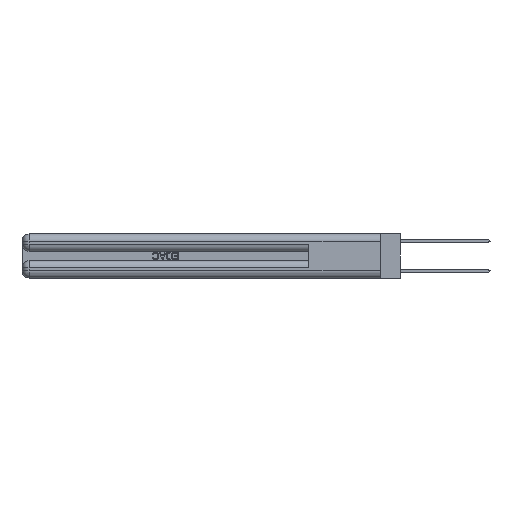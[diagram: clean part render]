
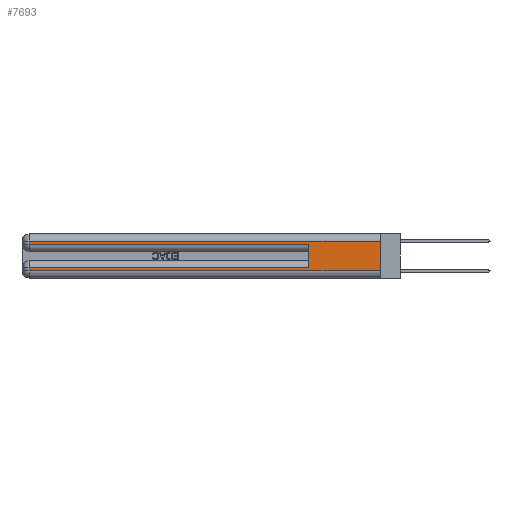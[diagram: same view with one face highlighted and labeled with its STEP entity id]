
A CAD part, left-side view. The second image highlights one B-rep face of the part: STEP entity #7693.
In plain terms, the highlighted planar face has unit normal (-1, 0, 0).
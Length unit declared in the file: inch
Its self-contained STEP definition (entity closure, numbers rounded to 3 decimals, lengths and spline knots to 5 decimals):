
#2025 = DIRECTION ( 'NONE',  ( 0., 0., -1. ) ) ;
#2323 = ORIENTED_EDGE ( 'NONE', *, *, #17587, .T. ) ;
#2801 = VECTOR ( 'NONE', #30167, 39.37008 ) ;
#4082 = CARTESIAN_POINT ( 'NONE',  ( 0., 0., 0.37 ) ) ;
#4154 = LINE ( 'NONE', #16316, #6959 ) ;
#4185 = CARTESIAN_POINT ( 'NONE',  ( 0., 2.94, 0.31 ) ) ;
#5009 = CARTESIAN_POINT ( 'NONE',  ( 0., 0., 0.31 ) ) ;
#6556 = LINE ( 'NONE', #8616, #17655 ) ;
#6946 = CARTESIAN_POINT ( 'NONE',  ( 0., 2.94, 0.37 ) ) ;
#6959 = VECTOR ( 'NONE', #13792, 39.37008 ) ;
#7693 = ADVANCED_FACE ( 'NONE', ( #28511 ), #28042, .F. ) ;
#8075 = DIRECTION ( 'NONE',  ( 0., -1., 0. ) ) ;
#8616 = CARTESIAN_POINT ( 'NONE',  ( 0., 0., 0.085 ) ) ;
#8637 = VECTOR ( 'NONE', #30842, 39.37008 ) ;
#9933 = CARTESIAN_POINT ( 'NONE',  ( 0., 0., 0.37 ) ) ;
#10361 = EDGE_LOOP ( 'NONE', ( #27957, #25769, #2323, #22479, #22251, #14810, #10801, #22275 ) ) ;
#10647 = VERTEX_POINT ( 'NONE', #10751 ) ;
#10662 = CARTESIAN_POINT ( 'NONE',  ( 0., 0.6, 0.285 ) ) ;
#10751 = CARTESIAN_POINT ( 'NONE',  ( 0., 0., 0.06 ) ) ;
#10801 = ORIENTED_EDGE ( 'NONE', *, *, #30165, .T. ) ;
#10812 = LINE ( 'NONE', #22941, #2801 ) ;
#12422 = VECTOR ( 'NONE', #28984, 39.37008 ) ;
#12439 = EDGE_CURVE ( 'NONE', #19086, #18914, #20362, .T. ) ;
#12474 = VERTEX_POINT ( 'NONE', #21292 ) ;
#12610 = DIRECTION ( 'NONE',  ( 1., 0., 0. ) ) ;
#13792 = DIRECTION ( 'NONE',  ( 0., 1., 0. ) ) ;
#14315 = EDGE_CURVE ( 'NONE', #18334, #10647, #14336, .T. ) ;
#14336 = LINE ( 'NONE', #24078, #14545 ) ;
#14545 = VECTOR ( 'NONE', #29401, 39.37008 ) ;
#14810 = ORIENTED_EDGE ( 'NONE', *, *, #25008, .T. ) ;
#15724 = VERTEX_POINT ( 'NONE', #5009 ) ;
#16025 = CARTESIAN_POINT ( 'NONE',  ( 0., 2.94, 0.285 ) ) ;
#16177 = DIRECTION ( 'NONE',  ( 0., 1., 0. ) ) ;
#16316 = CARTESIAN_POINT ( 'NONE',  ( 0., 0., 0.31 ) ) ;
#16795 = VERTEX_POINT ( 'NONE', #28550 ) ;
#17587 = EDGE_CURVE ( 'NONE', #19138, #19086, #23912, .T. ) ;
#17655 = VECTOR ( 'NONE', #16177, 39.37008 ) ;
#18334 = VERTEX_POINT ( 'NONE', #30897 ) ;
#18914 = VERTEX_POINT ( 'NONE', #10662 ) ;
#19086 = VERTEX_POINT ( 'NONE', #16025 ) ;
#19138 = VERTEX_POINT ( 'NONE', #4185 ) ;
#19347 = CARTESIAN_POINT ( 'NONE',  ( 0., 2.94, 0.37 ) ) ;
#19397 = LINE ( 'NONE', #6946, #12422 ) ;
#19762 = VECTOR ( 'NONE', #8075, 39.37008 ) ;
#20362 = LINE ( 'NONE', #29636, #19762 ) ;
#21292 = CARTESIAN_POINT ( 'NONE',  ( 0., 2.94, 0.085 ) ) ;
#21790 = AXIS2_PLACEMENT_3D ( 'NONE', #4082, #12610, #29276 ) ;
#22251 = ORIENTED_EDGE ( 'NONE', *, *, #29697, .F. ) ;
#22275 = ORIENTED_EDGE ( 'NONE', *, *, #14315, .T. ) ;
#22479 = ORIENTED_EDGE ( 'NONE', *, *, #12439, .T. ) ;
#22941 = CARTESIAN_POINT ( 'NONE',  ( 0., 0.6, 0.145 ) ) ;
#23912 = LINE ( 'NONE', #19347, #8637 ) ;
#24078 = CARTESIAN_POINT ( 'NONE',  ( 0., 0., 0.06 ) ) ;
#24102 = LINE ( 'NONE', #9933, #29960 ) ;
#25008 = EDGE_CURVE ( 'NONE', #16795, #12474, #6556, .T. ) ;
#25769 = ORIENTED_EDGE ( 'NONE', *, *, #27906, .T. ) ;
#27906 = EDGE_CURVE ( 'NONE', #15724, #19138, #4154, .T. ) ;
#27957 = ORIENTED_EDGE ( 'NONE', *, *, #28826, .F. ) ;
#28042 = PLANE ( 'NONE',  #21790 ) ;
#28511 = FACE_OUTER_BOUND ( 'NONE', #10361, .T. ) ;
#28550 = CARTESIAN_POINT ( 'NONE',  ( 0., 0.6, 0.085 ) ) ;
#28826 = EDGE_CURVE ( 'NONE', #15724, #10647, #24102, .T. ) ;
#28984 = DIRECTION ( 'NONE',  ( 0., 0., -1. ) ) ;
#29276 = DIRECTION ( 'NONE',  ( 0., 0., -1. ) ) ;
#29401 = DIRECTION ( 'NONE',  ( 0., -1., 0. ) ) ;
#29636 = CARTESIAN_POINT ( 'NONE',  ( 0., 0., 0.285 ) ) ;
#29697 = EDGE_CURVE ( 'NONE', #16795, #18914, #10812, .T. ) ;
#29960 = VECTOR ( 'NONE', #2025, 39.37008 ) ;
#30165 = EDGE_CURVE ( 'NONE', #12474, #18334, #19397, .T. ) ;
#30167 = DIRECTION ( 'NONE',  ( 0., 0., 1. ) ) ;
#30842 = DIRECTION ( 'NONE',  ( 0., 0., -1. ) ) ;
#30897 = CARTESIAN_POINT ( 'NONE',  ( 0., 2.94, 0.06 ) ) ;
